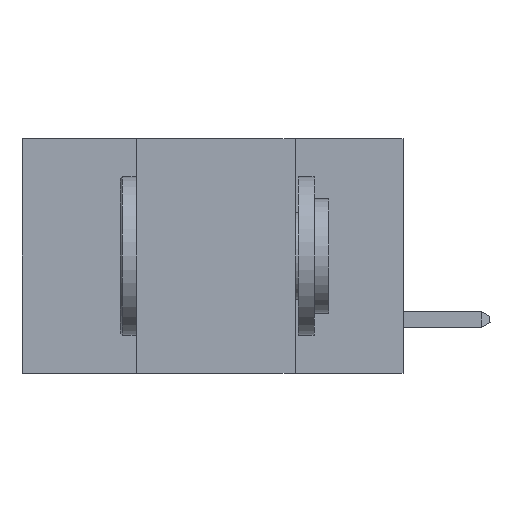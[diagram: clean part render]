
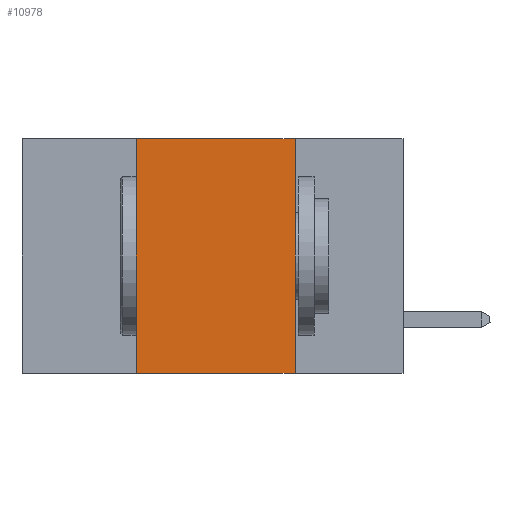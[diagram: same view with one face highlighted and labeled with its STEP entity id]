
A CAD part, left-side view. The second image highlights one B-rep face of the part: STEP entity #10978.
In plain terms, the highlighted planar face has unit normal (-1, 0, 0).
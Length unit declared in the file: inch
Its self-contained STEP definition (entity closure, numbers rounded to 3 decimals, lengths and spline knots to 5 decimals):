
#343 = CARTESIAN_POINT ( 'NONE',  ( 0., 0.17, 0. ) ) ;
#630 = EDGE_CURVE ( 'NONE', #4474, #7069, #4516, .T. ) ;
#1025 = CARTESIAN_POINT ( 'NONE',  ( 0., 0.42, 0. ) ) ;
#1167 = CARTESIAN_POINT ( 'NONE',  ( 0., 0.6, 0. ) ) ;
#1198 = ORIENTED_EDGE ( 'NONE', *, *, #14347, .T. ) ;
#1509 = DIRECTION ( 'NONE',  ( 0., -1., 0. ) ) ;
#1819 = VERTEX_POINT ( 'NONE', #14206 ) ;
#3134 = EDGE_CURVE ( 'NONE', #1819, #4474, #13701, .T. ) ;
#3504 = DIRECTION ( 'NONE',  ( 0., 0., 1. ) ) ;
#3876 = LINE ( 'NONE', #343, #6712 ) ;
#4474 = VERTEX_POINT ( 'NONE', #1025 ) ;
#4516 = LINE ( 'NONE', #5102, #5096 ) ;
#4715 = DIRECTION ( 'NONE',  ( 0., -1., 0. ) ) ;
#4809 = ORIENTED_EDGE ( 'NONE', *, *, #3134, .F. ) ;
#5029 = VERTEX_POINT ( 'NONE', #7349 ) ;
#5096 = VECTOR ( 'NONE', #1509, 39.37008 ) ;
#5102 = CARTESIAN_POINT ( 'NONE',  ( 0., 0.6, 0. ) ) ;
#5737 = CARTESIAN_POINT ( 'NONE',  ( 0., 0.17, 0. ) ) ;
#5886 = EDGE_LOOP ( 'NONE', ( #6108, #12902, #4809, #1198 ) ) ;
#6108 = ORIENTED_EDGE ( 'NONE', *, *, #12939, .F. ) ;
#6712 = VECTOR ( 'NONE', #9898, 39.37008 ) ;
#7069 = VERTEX_POINT ( 'NONE', #5737 ) ;
#7247 = DIRECTION ( 'NONE',  ( 1., 0., 0. ) ) ;
#7349 = CARTESIAN_POINT ( 'NONE',  ( 0., 0.17, -0.37 ) ) ;
#8393 = VECTOR ( 'NONE', #3504, 39.37008 ) ;
#9898 = DIRECTION ( 'NONE',  ( 0., 0., -1. ) ) ;
#10811 = DIRECTION ( 'NONE',  ( 0., 0., -1. ) ) ;
#10978 = ADVANCED_FACE ( 'NONE', ( #14233 ), #15655, .F. ) ;
#12079 = CARTESIAN_POINT ( 'NONE',  ( 0., 0.6, -0.37 ) ) ;
#12709 = LINE ( 'NONE', #12079, #13655 ) ;
#12902 = ORIENTED_EDGE ( 'NONE', *, *, #630, .F. ) ;
#12939 = EDGE_CURVE ( 'NONE', #7069, #5029, #3876, .T. ) ;
#12958 = AXIS2_PLACEMENT_3D ( 'NONE', #1167, #7247, #10811 ) ;
#13076 = CARTESIAN_POINT ( 'NONE',  ( 0., 0.42, 0. ) ) ;
#13655 = VECTOR ( 'NONE', #4715, 39.37008 ) ;
#13701 = LINE ( 'NONE', #13076, #8393 ) ;
#14206 = CARTESIAN_POINT ( 'NONE',  ( 0., 0.42, -0.37 ) ) ;
#14233 = FACE_OUTER_BOUND ( 'NONE', #5886, .T. ) ;
#14347 = EDGE_CURVE ( 'NONE', #1819, #5029, #12709, .T. ) ;
#15655 = PLANE ( 'NONE',  #12958 ) ;
